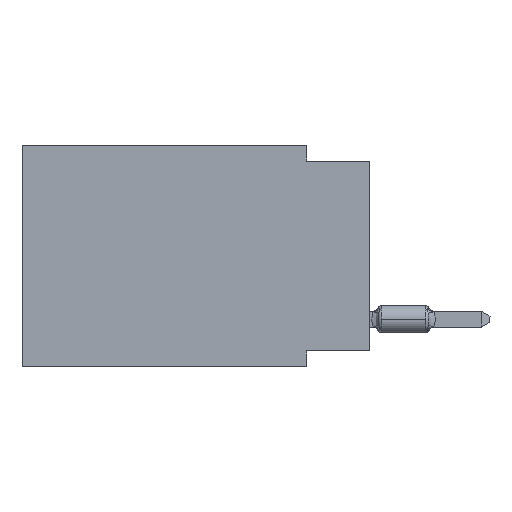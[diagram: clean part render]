
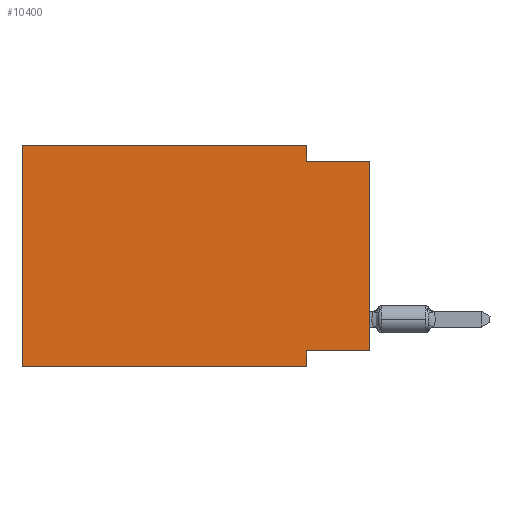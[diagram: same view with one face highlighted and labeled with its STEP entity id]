
A CAD part, left-side view. The second image highlights one B-rep face of the part: STEP entity #10400.
In plain terms, the highlighted planar face has unit normal (-1, 0, 0).
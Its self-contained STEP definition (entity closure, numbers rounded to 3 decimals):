
#306 = VECTOR ( 'NONE', #5539, 1000. ) ;
#927 = LINE ( 'NONE', #14181, #21531 ) ;
#1271 = CARTESIAN_POINT ( 'NONE',  ( 0., 2.54, 0. ) ) ;
#1332 = CARTESIAN_POINT ( 'NONE',  ( 0., 0., -8.255 ) ) ;
#1550 = DIRECTION ( 'NONE',  ( 0., -1., 0. ) ) ;
#1678 = LINE ( 'NONE', #15496, #17959 ) ;
#1706 = VECTOR ( 'NONE', #15650, 1000. ) ;
#1755 = VECTOR ( 'NONE', #11011, 1000. ) ;
#1865 = CARTESIAN_POINT ( 'NONE',  ( 0., 2.54, 0. ) ) ;
#1980 = EDGE_CURVE ( 'NONE', #19632, #14236, #927, .T. ) ;
#2000 = EDGE_CURVE ( 'NONE', #15495, #11475, #14299, .T. ) ;
#2466 = LINE ( 'NONE', #4172, #306 ) ;
#2561 = ORIENTED_EDGE ( 'NONE', *, *, #1980, .F. ) ;
#2761 = VERTEX_POINT ( 'NONE', #14466 ) ;
#3049 = ORIENTED_EDGE ( 'NONE', *, *, #2000, .T. ) ;
#3503 = PLANE ( 'NONE',  #12402 ) ;
#3618 = EDGE_LOOP ( 'NONE', ( #3049, #13995, #20194, #2561, #16955, #10468, #18146, #13094 ) ) ;
#4165 = EDGE_CURVE ( 'NONE', #2761, #11475, #10394, .T. ) ;
#4172 = CARTESIAN_POINT ( 'NONE',  ( 0., 13.97, 0. ) ) ;
#4283 = VECTOR ( 'NONE', #17002, 1000. ) ;
#4316 = CARTESIAN_POINT ( 'NONE',  ( 0., 2.54, -8.89 ) ) ;
#4961 = EDGE_CURVE ( 'NONE', #14236, #2761, #20618, .T. ) ;
#5187 = EDGE_CURVE ( 'NONE', #12750, #22374, #14618, .T. ) ;
#5354 = VECTOR ( 'NONE', #1550, 1000. ) ;
#5392 = CARTESIAN_POINT ( 'NONE',  ( 0., 13.97, 0. ) ) ;
#5428 = CARTESIAN_POINT ( 'NONE',  ( 0., 13.97, 0. ) ) ;
#5539 = DIRECTION ( 'NONE',  ( 0., 0., 1. ) ) ;
#5587 = DIRECTION ( 'NONE',  ( 0., -1., 0. ) ) ;
#6717 = CARTESIAN_POINT ( 'NONE',  ( 0., 2.54, -8.255 ) ) ;
#6890 = DIRECTION ( 'NONE',  ( 0., -1., 0. ) ) ;
#6899 = DIRECTION ( 'NONE',  ( 0., 0., -1. ) ) ;
#8586 = CARTESIAN_POINT ( 'NONE',  ( 0., 0., -0.635 ) ) ;
#8955 = CARTESIAN_POINT ( 'NONE',  ( 0., 13.97, -8.89 ) ) ;
#9096 = VERTEX_POINT ( 'NONE', #8955 ) ;
#10394 = LINE ( 'NONE', #8586, #5354 ) ;
#10400 = ADVANCED_FACE ( 'NONE', ( #20923 ), #3503, .F. ) ;
#10468 = ORIENTED_EDGE ( 'NONE', *, *, #19324, .T. ) ;
#11011 = DIRECTION ( 'NONE',  ( 0., 0., -1. ) ) ;
#11475 = VERTEX_POINT ( 'NONE', #11483 ) ;
#11483 = CARTESIAN_POINT ( 'NONE',  ( 0., 0., -0.635 ) ) ;
#12402 = AXIS2_PLACEMENT_3D ( 'NONE', #5428, #15277, #6899 ) ;
#12484 = CARTESIAN_POINT ( 'NONE',  ( 0., 0., -8.255 ) ) ;
#12750 = VERTEX_POINT ( 'NONE', #6717 ) ;
#13094 = ORIENTED_EDGE ( 'NONE', *, *, #21993, .F. ) ;
#13726 = LINE ( 'NONE', #12484, #1706 ) ;
#13995 = ORIENTED_EDGE ( 'NONE', *, *, #4165, .F. ) ;
#14181 = CARTESIAN_POINT ( 'NONE',  ( 0., 13.97, 0. ) ) ;
#14236 = VERTEX_POINT ( 'NONE', #1865 ) ;
#14299 = LINE ( 'NONE', #18687, #18651 ) ;
#14466 = CARTESIAN_POINT ( 'NONE',  ( 0., 2.54, -0.635 ) ) ;
#14618 = LINE ( 'NONE', #4316, #1755 ) ;
#15277 = DIRECTION ( 'NONE',  ( 1., 0., 0. ) ) ;
#15495 = VERTEX_POINT ( 'NONE', #1332 ) ;
#15496 = CARTESIAN_POINT ( 'NONE',  ( 0., 13.97, -8.89 ) ) ;
#15650 = DIRECTION ( 'NONE',  ( 0., 1., 0. ) ) ;
#16955 = ORIENTED_EDGE ( 'NONE', *, *, #21380, .F. ) ;
#17002 = DIRECTION ( 'NONE',  ( 0., 0., -1. ) ) ;
#17959 = VECTOR ( 'NONE', #6890, 1000. ) ;
#18146 = ORIENTED_EDGE ( 'NONE', *, *, #5187, .F. ) ;
#18651 = VECTOR ( 'NONE', #20382, 1000. ) ;
#18687 = CARTESIAN_POINT ( 'NONE',  ( 0., 0., 0. ) ) ;
#19324 = EDGE_CURVE ( 'NONE', #9096, #22374, #1678, .T. ) ;
#19632 = VERTEX_POINT ( 'NONE', #5392 ) ;
#20194 = ORIENTED_EDGE ( 'NONE', *, *, #4961, .F. ) ;
#20382 = DIRECTION ( 'NONE',  ( 0., 0., 1. ) ) ;
#20593 = CARTESIAN_POINT ( 'NONE',  ( 0., 2.54, -8.89 ) ) ;
#20618 = LINE ( 'NONE', #1271, #4283 ) ;
#20923 = FACE_OUTER_BOUND ( 'NONE', #3618, .T. ) ;
#21380 = EDGE_CURVE ( 'NONE', #9096, #19632, #2466, .T. ) ;
#21531 = VECTOR ( 'NONE', #5587, 1000. ) ;
#21993 = EDGE_CURVE ( 'NONE', #15495, #12750, #13726, .T. ) ;
#22374 = VERTEX_POINT ( 'NONE', #20593 ) ;
